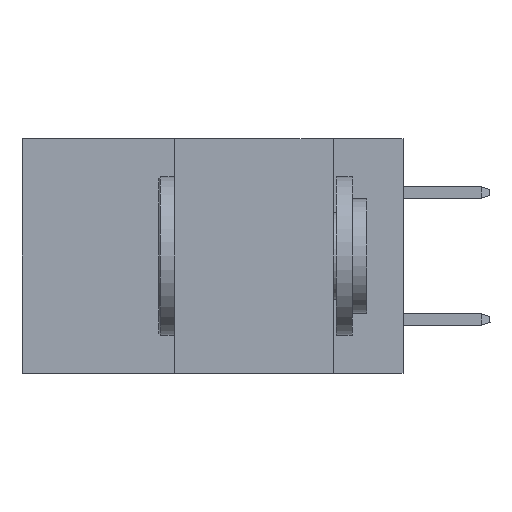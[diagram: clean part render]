
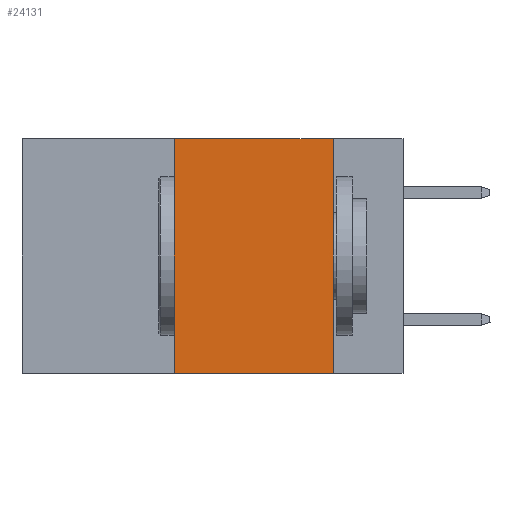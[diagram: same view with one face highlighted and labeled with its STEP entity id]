
A CAD part, left-side view. The second image highlights one B-rep face of the part: STEP entity #24131.
In plain terms, the highlighted planar face has unit normal (-1, 0, 0).
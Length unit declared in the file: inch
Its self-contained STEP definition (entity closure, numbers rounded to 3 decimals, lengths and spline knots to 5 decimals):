
#70 = LINE ( 'NONE', #29914, #26564 ) ;
#1131 = EDGE_CURVE ( 'NONE', #20959, #32333, #31230, .T. ) ;
#1274 = LINE ( 'NONE', #28621, #22980 ) ;
#1448 = AXIS2_PLACEMENT_3D ( 'NONE', #5322, #25434, #32349 ) ;
#2277 = VERTEX_POINT ( 'NONE', #18055 ) ;
#3373 = ORIENTED_EDGE ( 'NONE', *, *, #1131, .F. ) ;
#3734 = DIRECTION ( 'NONE',  ( 0., 0., -1. ) ) ;
#5322 = CARTESIAN_POINT ( 'NONE',  ( 0., 0.6, 0. ) ) ;
#8385 = EDGE_CURVE ( 'NONE', #15157, #20959, #1274, .T. ) ;
#8607 = ORIENTED_EDGE ( 'NONE', *, *, #8385, .F. ) ;
#8660 = CARTESIAN_POINT ( 'NONE',  ( 0., 0.11, 0. ) ) ;
#9703 = CARTESIAN_POINT ( 'NONE',  ( 0., 0.6, -0.37 ) ) ;
#10131 = DIRECTION ( 'NONE',  ( 0., 0., 1. ) ) ;
#11309 = DIRECTION ( 'NONE',  ( 0., -1., 0. ) ) ;
#12742 = PLANE ( 'NONE',  #1448 ) ;
#12922 = ORIENTED_EDGE ( 'NONE', *, *, #21169, .F. ) ;
#14315 = CARTESIAN_POINT ( 'NONE',  ( 0., 0.11, -0.37 ) ) ;
#14329 = VECTOR ( 'NONE', #3734, 39.37008 ) ;
#15157 = VERTEX_POINT ( 'NONE', #16565 ) ;
#15794 = ORIENTED_EDGE ( 'NONE', *, *, #24990, .T. ) ;
#16395 = CARTESIAN_POINT ( 'NONE',  ( 0., 0.11, 0. ) ) ;
#16565 = CARTESIAN_POINT ( 'NONE',  ( 0., 0.36, 0. ) ) ;
#16960 = LINE ( 'NONE', #9703, #27139 ) ;
#17194 = FACE_OUTER_BOUND ( 'NONE', #19992, .T. ) ;
#18055 = CARTESIAN_POINT ( 'NONE',  ( 0., 0.36, -0.37 ) ) ;
#19992 = EDGE_LOOP ( 'NONE', ( #3373, #8607, #12922, #15794 ) ) ;
#20959 = VERTEX_POINT ( 'NONE', #16395 ) ;
#21169 = EDGE_CURVE ( 'NONE', #2277, #15157, #70, .T. ) ;
#22980 = VECTOR ( 'NONE', #11309, 39.37008 ) ;
#24131 = ADVANCED_FACE ( 'NONE', ( #17194 ), #12742, .F. ) ;
#24990 = EDGE_CURVE ( 'NONE', #2277, #32333, #16960, .T. ) ;
#25434 = DIRECTION ( 'NONE',  ( 1., 0., 0. ) ) ;
#26564 = VECTOR ( 'NONE', #10131, 39.37008 ) ;
#27139 = VECTOR ( 'NONE', #27185, 39.37008 ) ;
#27185 = DIRECTION ( 'NONE',  ( 0., -1., 0. ) ) ;
#28621 = CARTESIAN_POINT ( 'NONE',  ( 0., 0.6, 0. ) ) ;
#29914 = CARTESIAN_POINT ( 'NONE',  ( 0., 0.36, 0. ) ) ;
#31230 = LINE ( 'NONE', #8660, #14329 ) ;
#32333 = VERTEX_POINT ( 'NONE', #14315 ) ;
#32349 = DIRECTION ( 'NONE',  ( 0., 0., -1. ) ) ;
